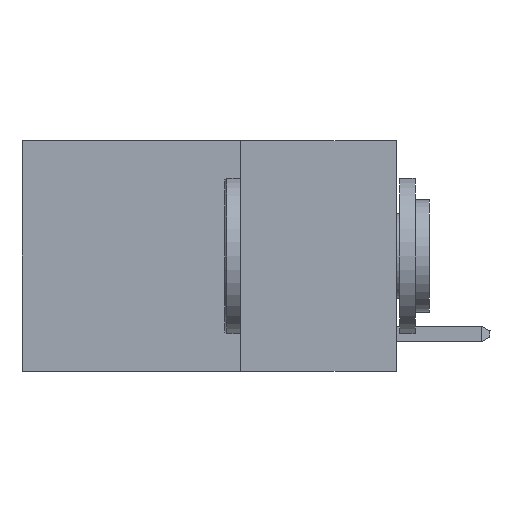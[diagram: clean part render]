
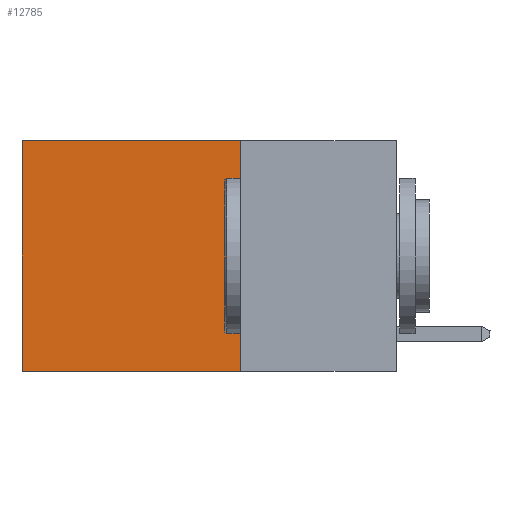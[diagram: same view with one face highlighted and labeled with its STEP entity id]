
A CAD part, left-side view. The second image highlights one B-rep face of the part: STEP entity #12785.
In plain terms, the highlighted planar face has unit normal (-1, 0, 0).
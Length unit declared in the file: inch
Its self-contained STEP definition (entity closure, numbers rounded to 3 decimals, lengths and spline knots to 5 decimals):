
#339 = VECTOR ( 'NONE', #4074, 39.37008 ) ;
#866 = DIRECTION ( 'NONE',  ( 0., 1., 0. ) ) ;
#1317 = VECTOR ( 'NONE', #8668, 39.37008 ) ;
#1410 = CARTESIAN_POINT ( 'NONE',  ( 0.2625, 0.25, -0.37 ) ) ;
#1561 = VERTEX_POINT ( 'NONE', #8094 ) ;
#2094 = CARTESIAN_POINT ( 'NONE',  ( 0.2625, 0.6, 0. ) ) ;
#2253 = ORIENTED_EDGE ( 'NONE', *, *, #12607, .T. ) ;
#2359 = AXIS2_PLACEMENT_3D ( 'NONE', #8893, #2827, #15161 ) ;
#2600 = VERTEX_POINT ( 'NONE', #2094 ) ;
#2640 = EDGE_CURVE ( 'NONE', #15116, #2600, #15479, .T. ) ;
#2827 = DIRECTION ( 'NONE',  ( 1., 0., 0. ) ) ;
#3245 = DIRECTION ( 'NONE',  ( 0., 0., -1. ) ) ;
#3550 = ORIENTED_EDGE ( 'NONE', *, *, #13422, .F. ) ;
#3674 = CARTESIAN_POINT ( 'NONE',  ( 0.2625, 0.25, -0.37 ) ) ;
#3970 = LINE ( 'NONE', #13348, #1317 ) ;
#4074 = DIRECTION ( 'NONE',  ( 0., 1., 0. ) ) ;
#4631 = EDGE_CURVE ( 'NONE', #7188, #1561, #5345, .T. ) ;
#5345 = LINE ( 'NONE', #1410, #339 ) ;
#7188 = VERTEX_POINT ( 'NONE', #3674 ) ;
#8094 = CARTESIAN_POINT ( 'NONE',  ( 0.2625, 0.6, -0.37 ) ) ;
#8668 = DIRECTION ( 'NONE',  ( 0., 0., -1. ) ) ;
#8813 = FACE_OUTER_BOUND ( 'NONE', #11222, .T. ) ;
#8893 = CARTESIAN_POINT ( 'NONE',  ( 0.2625, 0.25, 0. ) ) ;
#10188 = PLANE ( 'NONE',  #2359 ) ;
#10506 = VECTOR ( 'NONE', #3245, 39.37008 ) ;
#10757 = VECTOR ( 'NONE', #866, 39.37008 ) ;
#11222 = EDGE_LOOP ( 'NONE', ( #2253, #15890, #3550, #15828 ) ) ;
#11798 = CARTESIAN_POINT ( 'NONE',  ( 0.2625, 0.25, 0. ) ) ;
#12607 = EDGE_CURVE ( 'NONE', #2600, #1561, #15413, .T. ) ;
#12785 = ADVANCED_FACE ( 'NONE', ( #8813 ), #10188, .F. ) ;
#13348 = CARTESIAN_POINT ( 'NONE',  ( 0.2625, 0.25, 0. ) ) ;
#13422 = EDGE_CURVE ( 'NONE', #15116, #7188, #3970, .T. ) ;
#13999 = CARTESIAN_POINT ( 'NONE',  ( 0.2625, 0.25, 0. ) ) ;
#14266 = CARTESIAN_POINT ( 'NONE',  ( 0.2625, 0.6, 0. ) ) ;
#15116 = VERTEX_POINT ( 'NONE', #13999 ) ;
#15161 = DIRECTION ( 'NONE',  ( 0., 0., -1. ) ) ;
#15413 = LINE ( 'NONE', #14266, #10506 ) ;
#15479 = LINE ( 'NONE', #11798, #10757 ) ;
#15828 = ORIENTED_EDGE ( 'NONE', *, *, #2640, .T. ) ;
#15890 = ORIENTED_EDGE ( 'NONE', *, *, #4631, .F. ) ;
